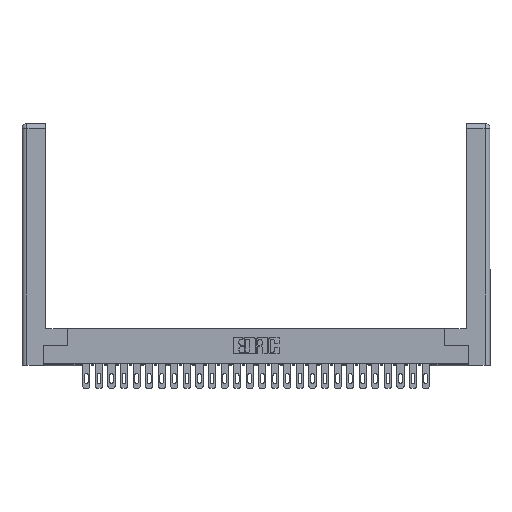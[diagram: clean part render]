
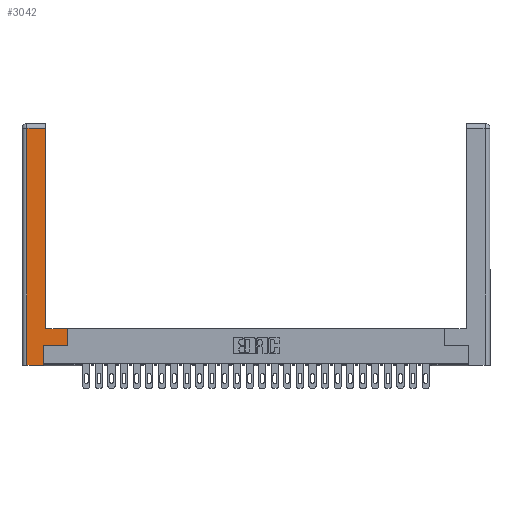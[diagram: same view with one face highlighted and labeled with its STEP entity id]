
A CAD part, top view. The second image highlights one B-rep face of the part: STEP entity #3042.
In plain terms, the highlighted planar face has unit normal (0, 0, 1).
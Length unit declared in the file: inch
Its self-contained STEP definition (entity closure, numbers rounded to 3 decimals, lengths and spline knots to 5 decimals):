
#143 = ORIENTED_EDGE ( 'NONE', *, *, #9901, .T. ) ;
#328 = CARTESIAN_POINT ( 'NONE',  ( 0.565, 0.45, 0. ) ) ;
#1127 = AXIS2_PLACEMENT_3D ( 'NONE', #28469, #15012, #12437 ) ;
#2183 = VECTOR ( 'NONE', #20801, 39.37008 ) ;
#3023 = EDGE_CURVE ( 'NONE', #25066, #34225, #20650, .T. ) ;
#3042 = ADVANCED_FACE ( 'NONE', ( #4377 ), #31262, .F. ) ;
#3311 = EDGE_CURVE ( 'NONE', #24132, #20802, #16835, .T. ) ;
#3490 = VERTEX_POINT ( 'NONE', #328 ) ;
#4377 = FACE_OUTER_BOUND ( 'NONE', #24618, .T. ) ;
#4654 = EDGE_CURVE ( 'NONE', #27013, #29914, #8881, .T. ) ;
#5587 = CARTESIAN_POINT ( 'NONE',  ( 0.295, 0.45, 0. ) ) ;
#5704 = ORIENTED_EDGE ( 'NONE', *, *, #26194, .T. ) ;
#5840 = VECTOR ( 'NONE', #14690, 39.37008 ) ;
#7063 = DIRECTION ( 'NONE',  ( 1., 0., 0. ) ) ;
#7353 = VECTOR ( 'NONE', #8885, 39.37008 ) ;
#7449 = LINE ( 'NONE', #17300, #18316 ) ;
#8881 = LINE ( 'NONE', #26569, #28574 ) ;
#8885 = DIRECTION ( 'NONE',  ( 0., 1., 0. ) ) ;
#9063 = CARTESIAN_POINT ( 'NONE',  ( 0.565, 0.45, 0. ) ) ;
#9901 = EDGE_CURVE ( 'NONE', #3490, #24132, #23573, .T. ) ;
#10413 = LINE ( 'NONE', #9063, #5840 ) ;
#10864 = CARTESIAN_POINT ( 'NONE',  ( 0.0615, 2.94, 0. ) ) ;
#11199 = DIRECTION ( 'NONE',  ( -1., 0., 0. ) ) ;
#11213 = VECTOR ( 'NONE', #11199, 39.37008 ) ;
#11684 = DIRECTION ( 'NONE',  ( 0., -1., 0. ) ) ;
#12327 = CARTESIAN_POINT ( 'NONE',  ( 0.565, 0.245, 0. ) ) ;
#12437 = DIRECTION ( 'NONE',  ( -1., 0., 0. ) ) ;
#13434 = CARTESIAN_POINT ( 'NONE',  ( 0.0615, 2.94, 0. ) ) ;
#13539 = VECTOR ( 'NONE', #19529, 39.37008 ) ;
#14402 = ORIENTED_EDGE ( 'NONE', *, *, #3023, .T. ) ;
#14690 = DIRECTION ( 'NONE',  ( 0., 1., 0. ) ) ;
#15012 = DIRECTION ( 'NONE',  ( 0., 0., -1. ) ) ;
#16835 = LINE ( 'NONE', #27515, #13539 ) ;
#17300 = CARTESIAN_POINT ( 'NONE',  ( 0.0615, 0., 0. ) ) ;
#17977 = CARTESIAN_POINT ( 'NONE',  ( 0.295, 2.94, 0. ) ) ;
#18316 = VECTOR ( 'NONE', #11684, 39.37008 ) ;
#18355 = DIRECTION ( 'NONE',  ( 1., 0., 0. ) ) ;
#18571 = VECTOR ( 'NONE', #7063, 39.37008 ) ;
#19235 = ORIENTED_EDGE ( 'NONE', *, *, #22912, .T. ) ;
#19529 = DIRECTION ( 'NONE',  ( 0., 1., 0. ) ) ;
#20182 = ORIENTED_EDGE ( 'NONE', *, *, #3311, .T. ) ;
#20650 = LINE ( 'NONE', #12327, #18571 ) ;
#20801 = DIRECTION ( 'NONE',  ( -1., 0., 0. ) ) ;
#20802 = VERTEX_POINT ( 'NONE', #17977 ) ;
#21375 = VERTEX_POINT ( 'NONE', #13434 ) ;
#22912 = EDGE_CURVE ( 'NONE', #20802, #21375, #27560, .T. ) ;
#23072 = EDGE_CURVE ( 'NONE', #21375, #27013, #7449, .T. ) ;
#23122 = ORIENTED_EDGE ( 'NONE', *, *, #23072, .T. ) ;
#23573 = LINE ( 'NONE', #32047, #2183 ) ;
#24132 = VERTEX_POINT ( 'NONE', #5587 ) ;
#24618 = EDGE_LOOP ( 'NONE', ( #20182, #19235, #23122, #28923, #30225, #14402, #5704, #143 ) ) ;
#25066 = VERTEX_POINT ( 'NONE', #25657 ) ;
#25657 = CARTESIAN_POINT ( 'NONE',  ( 0.265, 0.245, 0. ) ) ;
#26194 = EDGE_CURVE ( 'NONE', #34225, #3490, #10413, .T. ) ;
#26222 = CARTESIAN_POINT ( 'NONE',  ( 0.565, 0.245, 0. ) ) ;
#26569 = CARTESIAN_POINT ( 'NONE',  ( 0.265, 0., 0. ) ) ;
#27013 = VERTEX_POINT ( 'NONE', #34333 ) ;
#27515 = CARTESIAN_POINT ( 'NONE',  ( 0.295, 3., 0. ) ) ;
#27560 = LINE ( 'NONE', #10864, #11213 ) ;
#27642 = CARTESIAN_POINT ( 'NONE',  ( 0.265, 0.245, 0. ) ) ;
#28469 = CARTESIAN_POINT ( 'NONE',  ( 0., 0., 0. ) ) ;
#28574 = VECTOR ( 'NONE', #18355, 39.37008 ) ;
#28901 = CARTESIAN_POINT ( 'NONE',  ( 0.265, 0., 0. ) ) ;
#28919 = EDGE_CURVE ( 'NONE', #29914, #25066, #31614, .T. ) ;
#28923 = ORIENTED_EDGE ( 'NONE', *, *, #4654, .T. ) ;
#29914 = VERTEX_POINT ( 'NONE', #28901 ) ;
#30225 = ORIENTED_EDGE ( 'NONE', *, *, #28919, .T. ) ;
#31262 = PLANE ( 'NONE',  #1127 ) ;
#31614 = LINE ( 'NONE', #27642, #7353 ) ;
#32047 = CARTESIAN_POINT ( 'NONE',  ( 0.295, 0.45, 0. ) ) ;
#34225 = VERTEX_POINT ( 'NONE', #26222 ) ;
#34333 = CARTESIAN_POINT ( 'NONE',  ( 0.0615, 0., 0. ) ) ;
